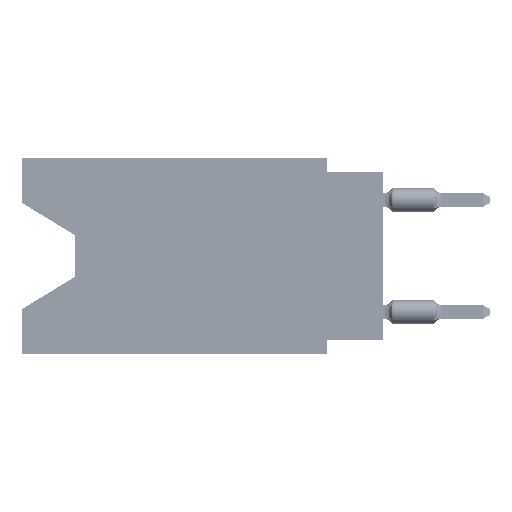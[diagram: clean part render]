
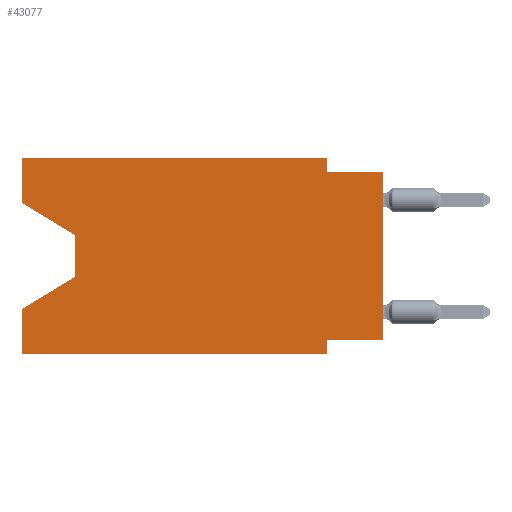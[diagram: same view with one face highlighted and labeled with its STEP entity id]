
A CAD part, left-side view. The second image highlights one B-rep face of the part: STEP entity #43077.
In plain terms, the highlighted planar face has unit normal (-1, 0, 0).
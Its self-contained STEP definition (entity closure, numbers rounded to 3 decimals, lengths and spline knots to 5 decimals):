
#3513 = VECTOR ( 'NONE', #82170, 39.37008 ) ;
#4228 = EDGE_CURVE ( 'NONE', #16790, #77928, #64974, .T. ) ;
#4294 = VECTOR ( 'NONE', #66615, 39.37008 ) ;
#6476 = VERTEX_POINT ( 'NONE', #82188 ) ;
#6839 = CARTESIAN_POINT ( 'NONE',  ( 0., 0.645, -0.08025 ) ) ;
#7006 = CARTESIAN_POINT ( 'NONE',  ( 0., 0., 0. ) ) ;
#7579 = LINE ( 'NONE', #31882, #98418 ) ;
#8116 = DIRECTION ( 'NONE',  ( 0., -1., 0. ) ) ;
#9294 = CARTESIAN_POINT ( 'NONE',  ( 0., 0.1, -0.325 ) ) ;
#11759 = CARTESIAN_POINT ( 'NONE',  ( 0., 0.55, -0.212 ) ) ;
#12525 = VECTOR ( 'NONE', #38687, 39.37008 ) ;
#13761 = CARTESIAN_POINT ( 'NONE',  ( 0., 0.645, 0. ) ) ;
#13941 = DIRECTION ( 'NONE',  ( 0., -0.855, -0.519 ) ) ;
#15013 = ORIENTED_EDGE ( 'NONE', *, *, #66680, .T. ) ;
#15259 = CARTESIAN_POINT ( 'NONE',  ( 0., 0.645, -0.08025 ) ) ;
#15890 = CARTESIAN_POINT ( 'NONE',  ( 0., 0.645, -0.35 ) ) ;
#16756 = LINE ( 'NONE', #85664, #34517 ) ;
#16782 = EDGE_CURVE ( 'NONE', #54415, #99324, #82674, .T. ) ;
#16790 = VERTEX_POINT ( 'NONE', #20350 ) ;
#18396 = EDGE_CURVE ( 'NONE', #35759, #53936, #76036, .T. ) ;
#18672 = VECTOR ( 'NONE', #74069, 39.37008 ) ;
#20350 = CARTESIAN_POINT ( 'NONE',  ( 0., 0.645, -0.35 ) ) ;
#22850 = DIRECTION ( 'NONE',  ( 0., 0., 1. ) ) ;
#26468 = CARTESIAN_POINT ( 'NONE',  ( 0., 0.645, 0. ) ) ;
#28018 = EDGE_CURVE ( 'NONE', #80246, #6476, #51423, .T. ) ;
#30466 = EDGE_CURVE ( 'NONE', #80246, #54415, #97133, .T. ) ;
#31694 = VERTEX_POINT ( 'NONE', #83002 ) ;
#31882 = CARTESIAN_POINT ( 'NONE',  ( 0., 0., -0.325 ) ) ;
#34009 = CARTESIAN_POINT ( 'NONE',  ( 0., 0.645, 0. ) ) ;
#34517 = VECTOR ( 'NONE', #39544, 39.37008 ) ;
#35681 = CARTESIAN_POINT ( 'NONE',  ( 0., 0.55, -0.138 ) ) ;
#35759 = VERTEX_POINT ( 'NONE', #94209 ) ;
#37998 = CARTESIAN_POINT ( 'NONE',  ( 0., 0., -0.025 ) ) ;
#38558 = CARTESIAN_POINT ( 'NONE',  ( 0., 0.645, 0. ) ) ;
#38687 = DIRECTION ( 'NONE',  ( 0., -1., 0. ) ) ;
#39544 = DIRECTION ( 'NONE',  ( 0., 0., -1. ) ) ;
#40198 = VECTOR ( 'NONE', #43947, 39.37008 ) ;
#40604 = DIRECTION ( 'NONE',  ( 0., 0., -1. ) ) ;
#42036 = AXIS2_PLACEMENT_3D ( 'NONE', #34009, #48711, #40604 ) ;
#43077 = ADVANCED_FACE ( 'NONE', ( #64424 ), #95828, .F. ) ;
#43947 = DIRECTION ( 'NONE',  ( 0., 0., 1. ) ) ;
#48711 = DIRECTION ( 'NONE',  ( 1., 0., 0. ) ) ;
#48832 = ORIENTED_EDGE ( 'NONE', *, *, #4228, .F. ) ;
#51423 = LINE ( 'NONE', #6839, #56403 ) ;
#51766 = VECTOR ( 'NONE', #22850, 39.37008 ) ;
#53088 = DIRECTION ( 'NONE',  ( 0., 0., 1. ) ) ;
#53936 = VERTEX_POINT ( 'NONE', #84297 ) ;
#54350 = CARTESIAN_POINT ( 'NONE',  ( 0., 0.1, 0. ) ) ;
#54357 = ORIENTED_EDGE ( 'NONE', *, *, #93750, .F. ) ;
#54415 = VERTEX_POINT ( 'NONE', #38558 ) ;
#55271 = EDGE_CURVE ( 'NONE', #16790, #83826, #85313, .T. ) ;
#56080 = EDGE_CURVE ( 'NONE', #31694, #72569, #7579, .T. ) ;
#56403 = VECTOR ( 'NONE', #13941, 39.37008 ) ;
#56861 = ORIENTED_EDGE ( 'NONE', *, *, #30466, .F. ) ;
#59012 = LINE ( 'NONE', #35681, #4294 ) ;
#60525 = EDGE_LOOP ( 'NONE', ( #93041, #79240, #15013, #48832, #92743, #72226, #99199, #63452, #81230, #54357, #74287, #56861 ) ) ;
#62522 = EDGE_CURVE ( 'NONE', #72569, #83826, #16756, .T. ) ;
#63452 = ORIENTED_EDGE ( 'NONE', *, *, #98351, .T. ) ;
#64424 = FACE_OUTER_BOUND ( 'NONE', #60525, .T. ) ;
#64974 = LINE ( 'NONE', #26468, #51766 ) ;
#66615 = DIRECTION ( 'NONE',  ( 0., 0., -1. ) ) ;
#66680 = EDGE_CURVE ( 'NONE', #86698, #77928, #90271, .T. ) ;
#67524 = EDGE_CURVE ( 'NONE', #6476, #86698, #59012, .T. ) ;
#68894 = DIRECTION ( 'NONE',  ( 0., 1., 0. ) ) ;
#72158 = DIRECTION ( 'NONE',  ( 0., 0., -1. ) ) ;
#72226 = ORIENTED_EDGE ( 'NONE', *, *, #62522, .F. ) ;
#72569 = VERTEX_POINT ( 'NONE', #9294 ) ;
#74069 = DIRECTION ( 'NONE',  ( 0., 0.855, -0.519 ) ) ;
#74287 = ORIENTED_EDGE ( 'NONE', *, *, #16782, .F. ) ;
#75162 = VECTOR ( 'NONE', #72158, 39.37008 ) ;
#76036 = LINE ( 'NONE', #37998, #89502 ) ;
#77680 = CARTESIAN_POINT ( 'NONE',  ( 0., 0.55, -0.212 ) ) ;
#77928 = VERTEX_POINT ( 'NONE', #80907 ) ;
#79240 = ORIENTED_EDGE ( 'NONE', *, *, #67524, .T. ) ;
#80246 = VERTEX_POINT ( 'NONE', #15259 ) ;
#80907 = CARTESIAN_POINT ( 'NONE',  ( 0., 0.645, -0.26975 ) ) ;
#81230 = ORIENTED_EDGE ( 'NONE', *, *, #18396, .F. ) ;
#81279 = CARTESIAN_POINT ( 'NONE',  ( 0., 0.1, 0. ) ) ;
#82170 = DIRECTION ( 'NONE',  ( 0., -1., 0. ) ) ;
#82188 = CARTESIAN_POINT ( 'NONE',  ( 0., 0.55, -0.138 ) ) ;
#82674 = LINE ( 'NONE', #13761, #3513 ) ;
#82986 = CARTESIAN_POINT ( 'NONE',  ( 0., 0.645, 0. ) ) ;
#83002 = CARTESIAN_POINT ( 'NONE',  ( 0., 0., -0.325 ) ) ;
#83826 = VERTEX_POINT ( 'NONE', #84669 ) ;
#84297 = CARTESIAN_POINT ( 'NONE',  ( 0., 0., -0.025 ) ) ;
#84507 = LINE ( 'NONE', #7006, #90796 ) ;
#84669 = CARTESIAN_POINT ( 'NONE',  ( 0., 0.1, -0.35 ) ) ;
#85313 = LINE ( 'NONE', #15890, #12525 ) ;
#85664 = CARTESIAN_POINT ( 'NONE',  ( 0., 0.1, -0.35 ) ) ;
#86698 = VERTEX_POINT ( 'NONE', #77680 ) ;
#86845 = LINE ( 'NONE', #81279, #75162 ) ;
#89502 = VECTOR ( 'NONE', #8116, 39.37008 ) ;
#90271 = LINE ( 'NONE', #11759, #18672 ) ;
#90796 = VECTOR ( 'NONE', #53088, 39.37008 ) ;
#92743 = ORIENTED_EDGE ( 'NONE', *, *, #55271, .T. ) ;
#93041 = ORIENTED_EDGE ( 'NONE', *, *, #28018, .T. ) ;
#93750 = EDGE_CURVE ( 'NONE', #99324, #35759, #86845, .T. ) ;
#94209 = CARTESIAN_POINT ( 'NONE',  ( 0., 0.1, -0.025 ) ) ;
#95828 = PLANE ( 'NONE',  #42036 ) ;
#97133 = LINE ( 'NONE', #82986, #40198 ) ;
#98351 = EDGE_CURVE ( 'NONE', #31694, #53936, #84507, .T. ) ;
#98418 = VECTOR ( 'NONE', #68894, 39.37008 ) ;
#99199 = ORIENTED_EDGE ( 'NONE', *, *, #56080, .F. ) ;
#99324 = VERTEX_POINT ( 'NONE', #54350 ) ;
